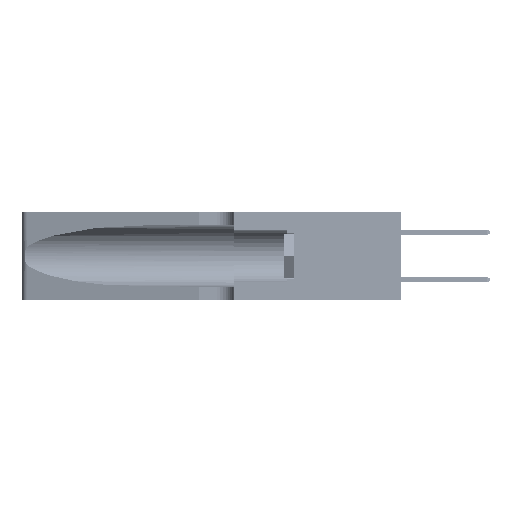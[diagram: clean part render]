
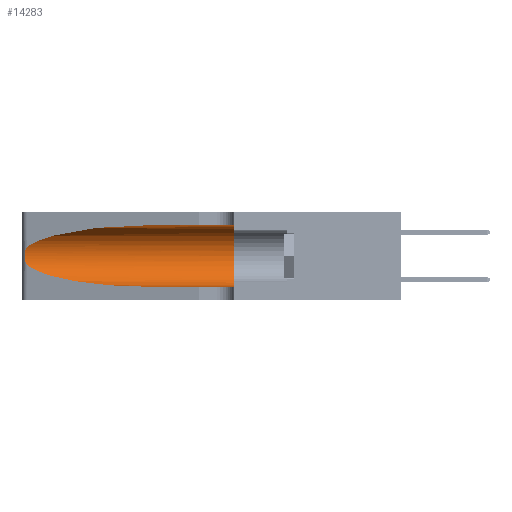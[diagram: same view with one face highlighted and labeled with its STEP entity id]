
A CAD part, left-side view. The second image highlights one B-rep face of the part: STEP entity #14283.
In plain terms, the highlighted cylindrical face has radius 3.308 mm (diameter 6.617 mm), a partial arc.
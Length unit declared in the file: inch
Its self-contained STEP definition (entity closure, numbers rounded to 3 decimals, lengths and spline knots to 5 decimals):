
#304 = CARTESIAN_POINT ( 'NONE',  ( 0.25787, 1.23484, 0.2124 ) ) ;
#738 = DIRECTION ( 'NONE',  ( 0., -1., 0. ) ) ;
#2925 = CARTESIAN_POINT ( 'NONE',  ( 0.1305, 1.61858, 0.31525 ) ) ;
#4459 = CARTESIAN_POINT ( 'NONE',  ( 0.26018, 1.23835, 0.19895 ) ) ;
#6218 = VERTEX_POINT ( 'NONE', #37285 ) ;
#6389 = VERTEX_POINT ( 'NONE', #47115 ) ;
#7230 = CARTESIAN_POINT ( 'NONE',  ( 0.25487, 1.22718, 0.22369 ) ) ;
#8515 = CARTESIAN_POINT ( 'NONE',  ( 0.26075, 1.23896, 0.178 ) ) ;
#9470 = ORIENTED_EDGE ( 'NONE', *, *, #18179, .T. ) ;
#10234 = ORIENTED_EDGE ( 'NONE', *, *, #31325, .F. ) ;
#12600 = CARTESIAN_POINT ( 'NONE',  ( 0.25856, 1.23593, 0.16098 ) ) ;
#12784 = CARTESIAN_POINT ( 'NONE',  ( 0.18966, 0.96281, 0.05475 ) ) ;
#13458 = EDGE_CURVE ( 'NONE', #6218, #26359, #38590, .T. ) ;
#13482 = CARTESIAN_POINT ( 'NONE',  ( 0.1305, 0.35, 0.05475 ) ) ;
#13568 = CARTESIAN_POINT ( 'NONE',  ( 0.18966, 0.96281, 0.31525 ) ) ;
#14145 = EDGE_CURVE ( 'NONE', #26359, #18313, #33697, .T. ) ;
#14283 = ADVANCED_FACE ( 'NONE', ( #38098 ), #16686, .F. ) ;
#15283 = CARTESIAN_POINT ( 'NONE',  ( 0.1305, 0.72297, 0.05475 ) ) ;
#15813 = VERTEX_POINT ( 'NONE', #7230 ) ;
#16653 = CARTESIAN_POINT ( 'NONE',  ( 0.25639, 1.23186, 0.15144 ) ) ;
#16686 = CYLINDRICAL_SURFACE ( 'NONE', #50559, 0.13025 ) ;
#17416 = DIRECTION ( 'NONE',  ( 0., 1., 0. ) ) ;
#17457 = CARTESIAN_POINT ( 'NONE',  ( 0.1305, 0.72297, 0.31525 ) ) ;
#17611 = DIRECTION ( 'NONE',  ( 0., -1., 0. ) ) ;
#17615 = CARTESIAN_POINT ( 'NONE',  ( 0.1305, 0.72297, 0.31525 ) ) ;
#17742 = ORIENTED_EDGE ( 'NONE', *, *, #38451, .F. ) ;
#18179 = EDGE_CURVE ( 'NONE', #15813, #6218, #29202, .T. ) ;
#18266 = CIRCLE ( 'NONE', #51967, 0.13025 ) ;
#18313 = VERTEX_POINT ( 'NONE', #13482 ) ;
#19566 = EDGE_CURVE ( 'NONE', #23099, #15813, #19869, .T. ) ;
#19869 =( BOUNDED_CURVE ( )  B_SPLINE_CURVE ( 3, ( #17615, #13568, #21640, #49756 ),
 .UNSPECIFIED., .F., .T. ) 
 B_SPLINE_CURVE_WITH_KNOTS ( ( 4, 4 ),
 ( 1.5708, 2.84003 ),
 .UNSPECIFIED. ) 
 CURVE ( )  GEOMETRIC_REPRESENTATION_ITEM ( )  RATIONAL_B_SPLINE_CURVE ( ( 1., 0.87, 0.87, 1. ) ) 
 REPRESENTATION_ITEM ( '' )  );
#20523 = CARTESIAN_POINT ( 'NONE',  ( 0.25487, 1.22718, 0.22369 ) ) ;
#20700 = CARTESIAN_POINT ( 'NONE',  ( 0.25487, 1.22718, 0.14631 ) ) ;
#21636 = CARTESIAN_POINT ( 'NONE',  ( 0.1305, 1.61858, 0.185 ) ) ;
#21640 = CARTESIAN_POINT ( 'NONE',  ( 0.2373, 1.15595, 0.28018 ) ) ;
#22978 = VECTOR ( 'NONE', #738, 39.37008 ) ;
#23099 = VERTEX_POINT ( 'NONE', #17457 ) ;
#24555 = CARTESIAN_POINT ( 'NONE',  ( 0.25639, 1.23184, 0.21858 ) ) ;
#25135 = VECTOR ( 'NONE', #39252, 39.37008 ) ;
#26359 = VERTEX_POINT ( 'NONE', #15283 ) ;
#28607 = CARTESIAN_POINT ( 'NONE',  ( 0.25854, 1.2359, 0.20912 ) ) ;
#28993 = ORIENTED_EDGE ( 'NONE', *, *, #19566, .T. ) ;
#29202 = B_SPLINE_CURVE_WITH_KNOTS ( 'NONE', 3,
 ( #20523, #40574, #24555, #304, #28607, #4459, #32643, #8515, #36718, #12600, #40754, #16653, #44775, #20700 ),
 .UNSPECIFIED., .F., .F.,
 ( 4, 2, 2, 2, 2, 2, 4 ),
 ( 0., 0.00027, 0.00053, 0.00107, 0.0016, 0.00187, 0.00214 ),
 .UNSPECIFIED. ) ;
#31325 = EDGE_CURVE ( 'NONE', #23099, #6389, #35886, .T. ) ;
#32643 = CARTESIAN_POINT ( 'NONE',  ( 0.26075, 1.23896, 0.19203 ) ) ;
#32834 = CARTESIAN_POINT ( 'NONE',  ( 0.25487, 1.22718, 0.14631 ) ) ;
#32886 = CARTESIAN_POINT ( 'NONE',  ( 0.1305, 1.61858, 0.05475 ) ) ;
#33697 = LINE ( 'NONE', #32886, #22978 ) ;
#35427 = ORIENTED_EDGE ( 'NONE', *, *, #14145, .T. ) ;
#35886 = LINE ( 'NONE', #2925, #25135 ) ;
#36718 = CARTESIAN_POINT ( 'NONE',  ( 0.26017, 1.23833, 0.17102 ) ) ;
#36913 = CARTESIAN_POINT ( 'NONE',  ( 0.2373, 1.15595, 0.08982 ) ) ;
#37285 = CARTESIAN_POINT ( 'NONE',  ( 0.25487, 1.22718, 0.14631 ) ) ;
#38098 = FACE_OUTER_BOUND ( 'NONE', #40830, .T. ) ;
#38451 = EDGE_CURVE ( 'NONE', #6389, #18313, #18266, .T. ) ;
#38590 =( BOUNDED_CURVE ( )  B_SPLINE_CURVE ( 3, ( #32834, #36913, #12784, #40947 ),
 .UNSPECIFIED., .F., .T. ) 
 B_SPLINE_CURVE_WITH_KNOTS ( ( 4, 4 ),
 ( 3.44316, 4.71239 ),
 .UNSPECIFIED. ) 
 CURVE ( )  GEOMETRIC_REPRESENTATION_ITEM ( )  RATIONAL_B_SPLINE_CURVE ( ( 1., 0.87, 0.87, 1. ) ) 
 REPRESENTATION_ITEM ( '' )  );
#39252 = DIRECTION ( 'NONE',  ( 0., -1., 0. ) ) ;
#40574 = CARTESIAN_POINT ( 'NONE',  ( 0.25555, 1.22994, 0.2215 ) ) ;
#40754 = CARTESIAN_POINT ( 'NONE',  ( 0.25789, 1.23486, 0.15765 ) ) ;
#40830 = EDGE_LOOP ( 'NONE', ( #28993, #9470, #42305, #35427, #17742, #10234 ) ) ;
#40947 = CARTESIAN_POINT ( 'NONE',  ( 0.1305, 0.72297, 0.05475 ) ) ;
#41519 = CARTESIAN_POINT ( 'NONE',  ( 0.1305, 0.35, 0.185 ) ) ;
#42305 = ORIENTED_EDGE ( 'NONE', *, *, #13458, .T. ) ;
#44775 = CARTESIAN_POINT ( 'NONE',  ( 0.25555, 1.22993, 0.14849 ) ) ;
#45531 = DIRECTION ( 'NONE',  ( 0., 0., 1. ) ) ;
#45717 = DIRECTION ( 'NONE',  ( 0., 0., -1. ) ) ;
#47115 = CARTESIAN_POINT ( 'NONE',  ( 0.1305, 0.35, 0.31525 ) ) ;
#49756 = CARTESIAN_POINT ( 'NONE',  ( 0.25487, 1.22718, 0.22369 ) ) ;
#50559 = AXIS2_PLACEMENT_3D ( 'NONE', #21636, #17611, #45717 ) ;
#51967 = AXIS2_PLACEMENT_3D ( 'NONE', #41519, #17416, #45531 ) ;
